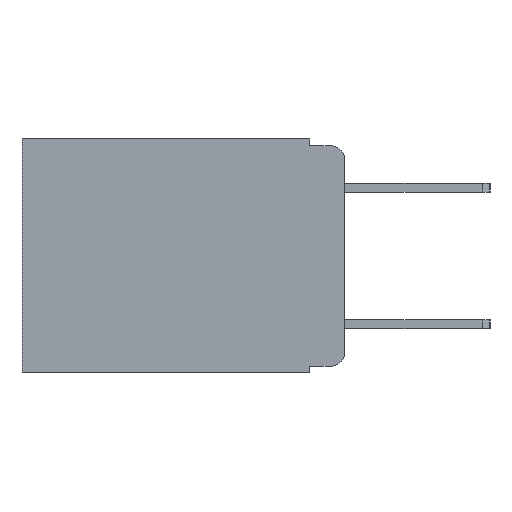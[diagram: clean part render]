
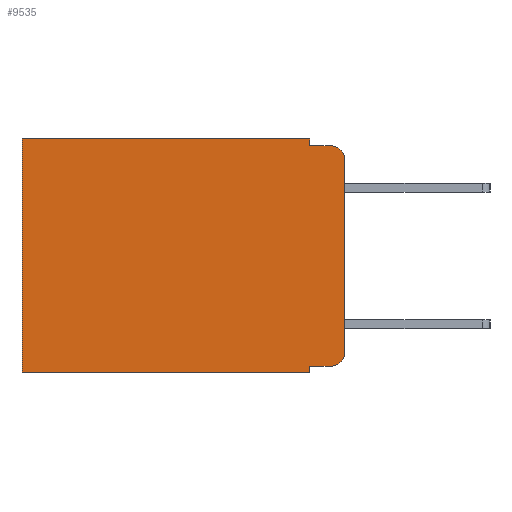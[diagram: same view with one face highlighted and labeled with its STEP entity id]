
A CAD part, left-side view. The second image highlights one B-rep face of the part: STEP entity #9535.
In plain terms, the highlighted planar face has unit normal (-1, 0, 0).
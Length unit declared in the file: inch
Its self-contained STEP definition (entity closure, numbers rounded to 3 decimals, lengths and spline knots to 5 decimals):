
#462 = AXIS2_PLACEMENT_3D ( 'NONE', #5130, #14650, #6482 ) ;
#609 = EDGE_CURVE ( 'NONE', #7307, #7330, #16932, .T. ) ;
#651 = ORIENTED_EDGE ( 'NONE', *, *, #16008, .T. ) ;
#790 = AXIS2_PLACEMENT_3D ( 'NONE', #6058, #2682, #12109 ) ;
#887 = LINE ( 'NONE', #5691, #7598 ) ;
#1157 = EDGE_CURVE ( 'NONE', #1191, #9456, #8850, .T. ) ;
#1191 = VERTEX_POINT ( 'NONE', #4404 ) ;
#1212 = ORIENTED_EDGE ( 'NONE', *, *, #10079, .T. ) ;
#1385 = CARTESIAN_POINT ( 'NONE',  ( 0.298, 0.051, -0.343 ) ) ;
#1477 = ORIENTED_EDGE ( 'NONE', *, *, #5841, .T. ) ;
#1567 = DIRECTION ( 'NONE',  ( 0., 0., -1. ) ) ;
#1652 = ORIENTED_EDGE ( 'NONE', *, *, #16224, .F. ) ;
#1822 = CARTESIAN_POINT ( 'NONE',  ( 0.298, 0.473, 0. ) ) ;
#1926 = CIRCLE ( 'NONE', #7266, 0.02 ) ;
#2013 = CARTESIAN_POINT ( 'NONE',  ( 0.298, 0.051, -0.333 ) ) ;
#2158 = ORIENTED_EDGE ( 'NONE', *, *, #17377, .F. ) ;
#2168 = VERTEX_POINT ( 'NONE', #11341 ) ;
#2568 = VERTEX_POINT ( 'NONE', #16744 ) ;
#2682 = DIRECTION ( 'NONE',  ( 1., 0., 0. ) ) ;
#2920 = VERTEX_POINT ( 'NONE', #1822 ) ;
#3073 = DIRECTION ( 'NONE',  ( -1., 0., 0. ) ) ;
#3343 = ORIENTED_EDGE ( 'NONE', *, *, #1157, .F. ) ;
#3841 = DIRECTION ( 'NONE',  ( 0., -1., 0. ) ) ;
#4404 = CARTESIAN_POINT ( 'NONE',  ( 0.298, 0., -0.03 ) ) ;
#5130 = CARTESIAN_POINT ( 'NONE',  ( 0.298, 0.02, -0.03 ) ) ;
#5146 = CARTESIAN_POINT ( 'NONE',  ( 0.298, 0.051, -0.333 ) ) ;
#5166 = CARTESIAN_POINT ( 'NONE',  ( 0.298, 0., -0.313 ) ) ;
#5497 = VECTOR ( 'NONE', #13321, 39.37008 ) ;
#5527 = ORIENTED_EDGE ( 'NONE', *, *, #609, .F. ) ;
#5543 = ORIENTED_EDGE ( 'NONE', *, *, #16806, .T. ) ;
#5691 = CARTESIAN_POINT ( 'NONE',  ( 0.298, 0.051, 0. ) ) ;
#5841 = EDGE_CURVE ( 'NONE', #2168, #2920, #12723, .T. ) ;
#6058 = CARTESIAN_POINT ( 'NONE',  ( 0.298, 0., 0. ) ) ;
#6204 = CARTESIAN_POINT ( 'NONE',  ( 0.298, 0., -0.343 ) ) ;
#6482 = DIRECTION ( 'NONE',  ( 0., 0., -1. ) ) ;
#6584 = EDGE_CURVE ( 'NONE', #2168, #2568, #887, .T. ) ;
#6629 = LINE ( 'NONE', #15083, #13879 ) ;
#7266 = AXIS2_PLACEMENT_3D ( 'NONE', #11142, #3073, #12524 ) ;
#7293 = DIRECTION ( 'NONE',  ( 0., 0., -1. ) ) ;
#7307 = VERTEX_POINT ( 'NONE', #1385 ) ;
#7330 = VERTEX_POINT ( 'NONE', #8090 ) ;
#7598 = VECTOR ( 'NONE', #7293, 39.37008 ) ;
#7903 = EDGE_CURVE ( 'NONE', #8156, #9456, #1926, .T. ) ;
#7940 = FACE_OUTER_BOUND ( 'NONE', #15378, .T. ) ;
#8090 = CARTESIAN_POINT ( 'NONE',  ( 0.298, 0.473, -0.343 ) ) ;
#8156 = VERTEX_POINT ( 'NONE', #14671 ) ;
#8850 = LINE ( 'NONE', #12412, #15665 ) ;
#9207 = LINE ( 'NONE', #16446, #12379 ) ;
#9361 = DIRECTION ( 'NONE',  ( 0., 0., -1. ) ) ;
#9424 = VECTOR ( 'NONE', #3841, 39.37008 ) ;
#9456 = VERTEX_POINT ( 'NONE', #5166 ) ;
#9535 = ADVANCED_FACE ( 'NONE', ( #7940 ), #17446, .F. ) ;
#10079 = EDGE_CURVE ( 'NONE', #15782, #8156, #13019, .T. ) ;
#11142 = CARTESIAN_POINT ( 'NONE',  ( 0.298, 0.02, -0.313 ) ) ;
#11341 = CARTESIAN_POINT ( 'NONE',  ( 0.298, 0.051, 0. ) ) ;
#11589 = DIRECTION ( 'NONE',  ( 0., 1., 0. ) ) ;
#11636 = CARTESIAN_POINT ( 'NONE',  ( 0.298, 0.02, -0.01 ) ) ;
#12109 = DIRECTION ( 'NONE',  ( 0., 0., -1. ) ) ;
#12117 = CARTESIAN_POINT ( 'NONE',  ( 0.298, 0.051, -0.01 ) ) ;
#12130 = LINE ( 'NONE', #12117, #15346 ) ;
#12255 = VERTEX_POINT ( 'NONE', #11636 ) ;
#12379 = VECTOR ( 'NONE', #1567, 39.37008 ) ;
#12412 = CARTESIAN_POINT ( 'NONE',  ( 0.298, 0., 0. ) ) ;
#12524 = DIRECTION ( 'NONE',  ( 0., 0., -1. ) ) ;
#12723 = LINE ( 'NONE', #13037, #5497 ) ;
#12785 = ORIENTED_EDGE ( 'NONE', *, *, #6584, .F. ) ;
#13019 = LINE ( 'NONE', #5146, #9424 ) ;
#13037 = CARTESIAN_POINT ( 'NONE',  ( 0.298, 0., 0. ) ) ;
#13321 = DIRECTION ( 'NONE',  ( 0., 1., 0. ) ) ;
#13332 = VECTOR ( 'NONE', #11589, 39.37008 ) ;
#13493 = DIRECTION ( 'NONE',  ( 0., -1., 0. ) ) ;
#13879 = VECTOR ( 'NONE', #16431, 39.37008 ) ;
#14650 = DIRECTION ( 'NONE',  ( -1., 0., 0. ) ) ;
#14671 = CARTESIAN_POINT ( 'NONE',  ( 0.298, 0.02, -0.333 ) ) ;
#15083 = CARTESIAN_POINT ( 'NONE',  ( 0.298, 0.473, 0. ) ) ;
#15346 = VECTOR ( 'NONE', #13493, 39.37008 ) ;
#15378 = EDGE_LOOP ( 'NONE', ( #3343, #651, #2158, #12785, #1477, #5543, #5527, #1652, #1212, #15984 ) ) ;
#15665 = VECTOR ( 'NONE', #9361, 39.37008 ) ;
#15782 = VERTEX_POINT ( 'NONE', #2013 ) ;
#15820 = CIRCLE ( 'NONE', #462, 0.02 ) ;
#15984 = ORIENTED_EDGE ( 'NONE', *, *, #7903, .T. ) ;
#16008 = EDGE_CURVE ( 'NONE', #1191, #12255, #15820, .T. ) ;
#16224 = EDGE_CURVE ( 'NONE', #15782, #7307, #9207, .T. ) ;
#16431 = DIRECTION ( 'NONE',  ( 0., 0., -1. ) ) ;
#16446 = CARTESIAN_POINT ( 'NONE',  ( 0.298, 0.051, 0. ) ) ;
#16744 = CARTESIAN_POINT ( 'NONE',  ( 0.298, 0.051, -0.01 ) ) ;
#16806 = EDGE_CURVE ( 'NONE', #2920, #7330, #6629, .T. ) ;
#16932 = LINE ( 'NONE', #6204, #13332 ) ;
#17377 = EDGE_CURVE ( 'NONE', #2568, #12255, #12130, .T. ) ;
#17446 = PLANE ( 'NONE',  #790 ) ;
